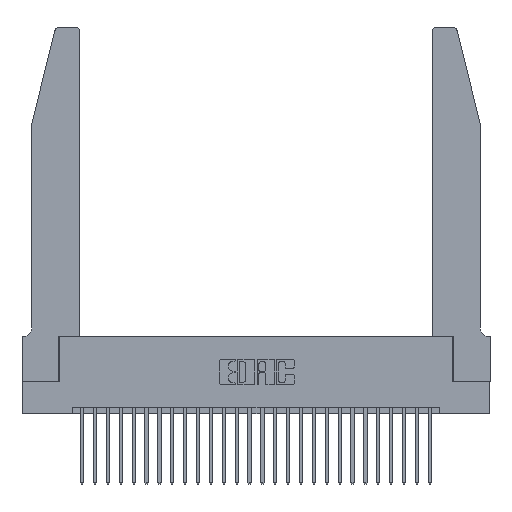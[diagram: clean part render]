
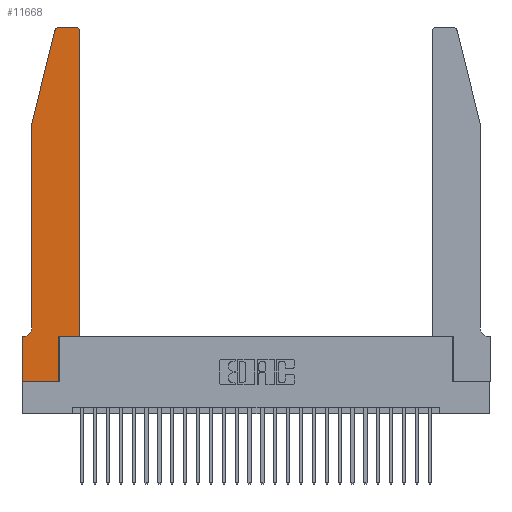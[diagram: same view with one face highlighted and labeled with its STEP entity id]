
A CAD part, top view. The second image highlights one B-rep face of the part: STEP entity #11668.
In plain terms, the highlighted planar face has unit normal (0, 0, 1).
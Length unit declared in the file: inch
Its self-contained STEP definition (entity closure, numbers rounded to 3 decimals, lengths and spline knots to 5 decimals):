
#333 = CARTESIAN_POINT ( 'NONE',  ( 0.284, 2.75, 0.37 ) ) ;
#344 = ORIENTED_EDGE ( 'NONE', *, *, #5128, .T. ) ;
#662 = CARTESIAN_POINT ( 'NONE',  ( 0.4505, 0.35, 0.37 ) ) ;
#724 = VERTEX_POINT ( 'NONE', #10554 ) ;
#1047 = DIRECTION ( 'NONE',  ( -1., 0., 0. ) ) ;
#1063 = ORIENTED_EDGE ( 'NONE', *, *, #28521, .T. ) ;
#1649 = CARTESIAN_POINT ( 'NONE',  ( 0.4505, 0.35, 0.37 ) ) ;
#1875 = DIRECTION ( 'NONE',  ( 0., 1., 0. ) ) ;
#2017 = LINE ( 'NONE', #1649, #12556 ) ;
#2670 = AXIS2_PLACEMENT_3D ( 'NONE', #18690, #5390, #20870 ) ;
#2821 = CARTESIAN_POINT ( 'NONE',  ( 0.0755, 2., 0.37 ) ) ;
#3284 = VERTEX_POINT ( 'NONE', #18066 ) ;
#3513 = EDGE_CURVE ( 'NONE', #12134, #11735, #14731, .T. ) ;
#3527 = ORIENTED_EDGE ( 'NONE', *, *, #19521, .T. ) ;
#3698 = CARTESIAN_POINT ( 'NONE',  ( 0., 0.35, 0.37 ) ) ;
#4040 = VECTOR ( 'NONE', #22824, 39.37008 ) ;
#4290 = DIRECTION ( 'NONE',  ( 0., -1., 0. ) ) ;
#4601 = ORIENTED_EDGE ( 'NONE', *, *, #13701, .T. ) ;
#5128 = EDGE_CURVE ( 'NONE', #11778, #3284, #6588, .T. ) ;
#5390 = DIRECTION ( 'NONE',  ( 0., 0., 1. ) ) ;
#5400 = LINE ( 'NONE', #2821, #9250 ) ;
#5412 = DIRECTION ( 'NONE',  ( 1., 0., 0. ) ) ;
#5437 = VECTOR ( 'NONE', #26915, 39.37008 ) ;
#5465 = VERTEX_POINT ( 'NONE', #25360 ) ;
#5901 = VERTEX_POINT ( 'NONE', #333 ) ;
#6434 = EDGE_CURVE ( 'NONE', #22854, #5901, #16607, .T. ) ;
#6588 = LINE ( 'NONE', #8701, #24177 ) ;
#7110 = AXIS2_PLACEMENT_3D ( 'NONE', #27516, #14513, #1047 ) ;
#7212 = EDGE_CURVE ( 'NONE', #5465, #22517, #10012, .T. ) ;
#7244 = VERTEX_POINT ( 'NONE', #662 ) ;
#7617 = EDGE_CURVE ( 'NONE', #20428, #7244, #23063, .T. ) ;
#8256 = DIRECTION ( 'NONE',  ( 1., 0., 0. ) ) ;
#8547 = CARTESIAN_POINT ( 'NONE',  ( 0.0055, 0.35, 0.37 ) ) ;
#8701 = CARTESIAN_POINT ( 'NONE',  ( 0.0755, 0.35, 0.37 ) ) ;
#8799 = VECTOR ( 'NONE', #5412, 39.37008 ) ;
#9186 = ORIENTED_EDGE ( 'NONE', *, *, #7617, .T. ) ;
#9250 = VECTOR ( 'NONE', #20610, 39.37008 ) ;
#9300 = EDGE_LOOP ( 'NONE', ( #19879, #26322, #3527, #21244, #10923, #344, #1063, #18866, #20229, #9186, #4601, #16481 ) ) ;
#9390 = CARTESIAN_POINT ( 'NONE',  ( 0.4505, 0.35, 0.37 ) ) ;
#10012 = LINE ( 'NONE', #16253, #4040 ) ;
#10358 = CIRCLE ( 'NONE', #2670, 0.03 ) ;
#10441 = CARTESIAN_POINT ( 'NONE',  ( 0.284, 2.72, 0.37 ) ) ;
#10460 = VERTEX_POINT ( 'NONE', #12983 ) ;
#10508 = EDGE_CURVE ( 'NONE', #11735, #20428, #16848, .T. ) ;
#10554 = CARTESIAN_POINT ( 'NONE',  ( 0.4505, 2.72, 0.37 ) ) ;
#10923 = ORIENTED_EDGE ( 'NONE', *, *, #28242, .T. ) ;
#11668 = ADVANCED_FACE ( 'NONE', ( #21949 ), #19265, .T. ) ;
#11735 = VERTEX_POINT ( 'NONE', #23825 ) ;
#11778 = VERTEX_POINT ( 'NONE', #8547 ) ;
#11929 = AXIS2_PLACEMENT_3D ( 'NONE', #10441, #25762, #12682 ) ;
#12134 = VERTEX_POINT ( 'NONE', #18562 ) ;
#12322 = CARTESIAN_POINT ( 'NONE',  ( 0.2865, 0.35, 0.37 ) ) ;
#12556 = VECTOR ( 'NONE', #19476, 39.37008 ) ;
#12682 = DIRECTION ( 'NONE',  ( 1., 0., 0. ) ) ;
#12953 = CIRCLE ( 'NONE', #7110, 0.07 ) ;
#12983 = CARTESIAN_POINT ( 'NONE',  ( 0.25487, 2.72718, 0.37 ) ) ;
#13270 = DIRECTION ( 'NONE',  ( -1., 0., 0. ) ) ;
#13701 = EDGE_CURVE ( 'NONE', #7244, #724, #2017, .T. ) ;
#14513 = DIRECTION ( 'NONE',  ( 0., 0., -1. ) ) ;
#14731 = LINE ( 'NONE', #25166, #8799 ) ;
#14804 = VECTOR ( 'NONE', #1875, 39.37008 ) ;
#15676 = EDGE_CURVE ( 'NONE', #724, #22854, #10358, .T. ) ;
#16253 = CARTESIAN_POINT ( 'NONE',  ( 0.0755, 2., 0.37 ) ) ;
#16481 = ORIENTED_EDGE ( 'NONE', *, *, #15676, .T. ) ;
#16607 = LINE ( 'NONE', #20095, #27473 ) ;
#16848 = LINE ( 'NONE', #17514, #14804 ) ;
#17514 = CARTESIAN_POINT ( 'NONE',  ( 0.2865, 0.35, 0.37 ) ) ;
#17644 = CARTESIAN_POINT ( 'NONE',  ( 0., 0., 0.37 ) ) ;
#17756 = LINE ( 'NONE', #17644, #22855 ) ;
#18066 = CARTESIAN_POINT ( 'NONE',  ( 0., 0.35, 0.37 ) ) ;
#18562 = CARTESIAN_POINT ( 'NONE',  ( 0., 0., 0.37 ) ) ;
#18690 = CARTESIAN_POINT ( 'NONE',  ( 0.4205, 2.72, 0.37 ) ) ;
#18866 = ORIENTED_EDGE ( 'NONE', *, *, #3513, .T. ) ;
#19265 = PLANE ( 'NONE',  #22697 ) ;
#19476 = DIRECTION ( 'NONE',  ( 0., 1., 0. ) ) ;
#19521 = EDGE_CURVE ( 'NONE', #10460, #5465, #5400, .T. ) ;
#19879 = ORIENTED_EDGE ( 'NONE', *, *, #6434, .T. ) ;
#20095 = CARTESIAN_POINT ( 'NONE',  ( 0.2605, 2.75, 0.37 ) ) ;
#20229 = ORIENTED_EDGE ( 'NONE', *, *, #10508, .T. ) ;
#20428 = VERTEX_POINT ( 'NONE', #12322 ) ;
#20610 = DIRECTION ( 'NONE',  ( -0.239, -0.971, 0. ) ) ;
#20870 = DIRECTION ( 'NONE',  ( 1., 0., 0. ) ) ;
#20973 = CARTESIAN_POINT ( 'NONE',  ( 0.4205, 2.75, 0.37 ) ) ;
#21244 = ORIENTED_EDGE ( 'NONE', *, *, #7212, .T. ) ;
#21455 = DIRECTION ( 'NONE',  ( 0., 0., 1. ) ) ;
#21875 = CARTESIAN_POINT ( 'NONE',  ( 0.0755, 0.42, 0.37 ) ) ;
#21949 = FACE_OUTER_BOUND ( 'NONE', #9300, .T. ) ;
#22302 = DIRECTION ( 'NONE',  ( -1., 0., 0. ) ) ;
#22517 = VERTEX_POINT ( 'NONE', #21875 ) ;
#22697 = AXIS2_PLACEMENT_3D ( 'NONE', #3698, #21455, #8256 ) ;
#22824 = DIRECTION ( 'NONE',  ( 0., -1., 0. ) ) ;
#22854 = VERTEX_POINT ( 'NONE', #20973 ) ;
#22855 = VECTOR ( 'NONE', #4290, 39.37008 ) ;
#23063 = LINE ( 'NONE', #9390, #5437 ) ;
#23825 = CARTESIAN_POINT ( 'NONE',  ( 0.2865, 0., 0.37 ) ) ;
#24177 = VECTOR ( 'NONE', #13270, 39.37008 ) ;
#25166 = CARTESIAN_POINT ( 'NONE',  ( 0., 0., 0.37 ) ) ;
#25360 = CARTESIAN_POINT ( 'NONE',  ( 0.0755, 2., 0.37 ) ) ;
#25762 = DIRECTION ( 'NONE',  ( 0., 0., 1. ) ) ;
#26240 = EDGE_CURVE ( 'NONE', #5901, #10460, #28370, .T. ) ;
#26322 = ORIENTED_EDGE ( 'NONE', *, *, #26240, .T. ) ;
#26915 = DIRECTION ( 'NONE',  ( 1., 0., 0. ) ) ;
#27473 = VECTOR ( 'NONE', #22302, 39.37008 ) ;
#27516 = CARTESIAN_POINT ( 'NONE',  ( 0.0055, 0.42, 0.37 ) ) ;
#28242 = EDGE_CURVE ( 'NONE', #22517, #11778, #12953, .T. ) ;
#28370 = CIRCLE ( 'NONE', #11929, 0.03 ) ;
#28521 = EDGE_CURVE ( 'NONE', #3284, #12134, #17756, .T. ) ;
